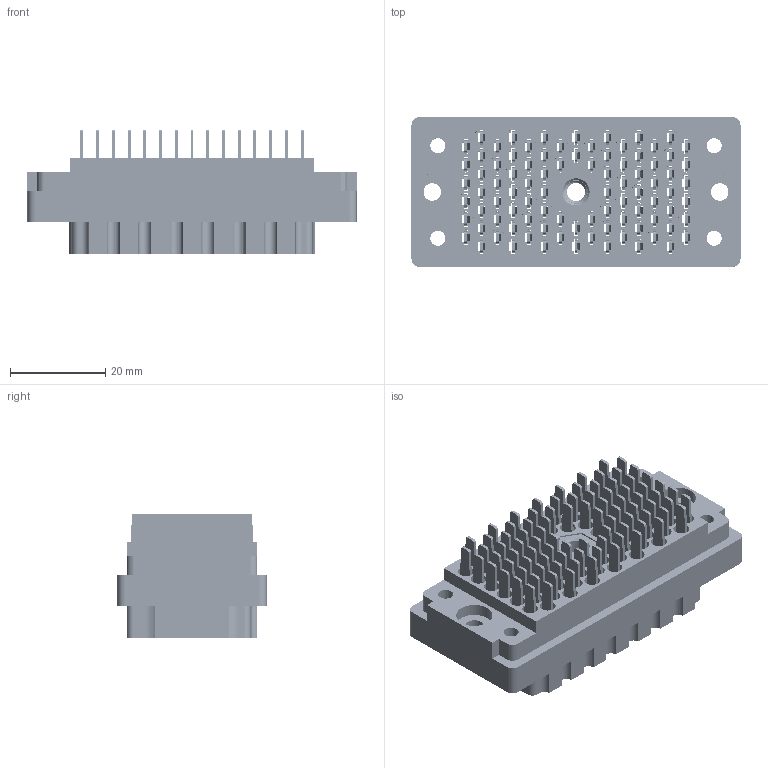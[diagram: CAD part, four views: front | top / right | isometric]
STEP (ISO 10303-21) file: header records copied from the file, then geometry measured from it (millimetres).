
FILE_DESCRIPTION (( 'STEP AP203' ), '1' );
FILE_NAME ('516-090-501-406.STEP', '2020-09-08T18:00:51', ( '' ), ( '' ), 'SwSTEP 2.0', 'SolidWorks 2020', '' );
FILE_SCHEMA (( 'CONFIG_CONTROL_DESIGN' ));
Length unit declared in the file: inch
Products named in the file (4): 516-292-001_501 Contact; 516-090-501-406; 516-252-095-100; 516 Part Receptacle_090
Assembly tree (93 placements, depth 2):
  516-090-501-406
    516 Part Receptacle_090
    516-292-001_501 Contact  x91
    516-252-095-100
Bounding box: 69.04 x 31.34 x 26.21 mm (x, y, z)
Volume: 23670.1 mm3; surface area: 46854.6 mm2
Topology: 93 solids, 93 shells, 8527 faces, 24775 edges, 16453 vertices
Faces by surface type: plane 5117, cylinder 2846, bspline 552, cone 12
Entity records: 74163 total; most frequent: CARTESIAN_POINT 14520, ORIENTED_EDGE 12110, DIRECTION 11770, EDGE_CURVE 6055, VECTOR 4438, LINE 4438, VERTEX_POINT 4033, AXIS2_PLACEMENT_3D 3666
